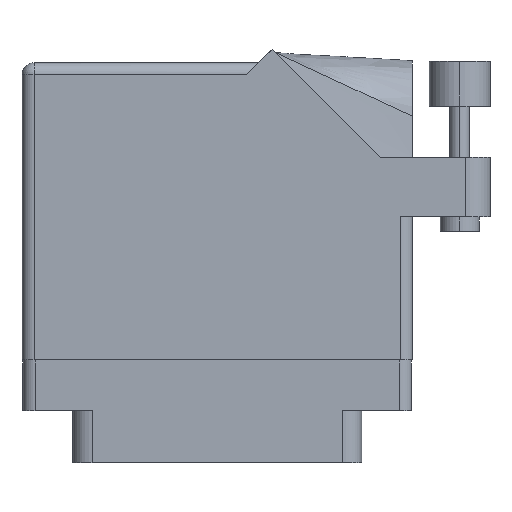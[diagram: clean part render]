
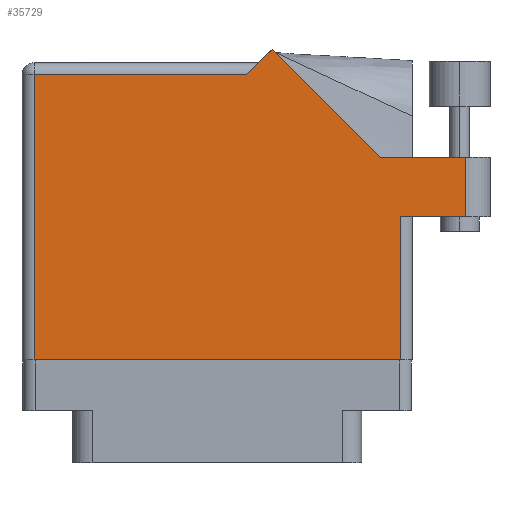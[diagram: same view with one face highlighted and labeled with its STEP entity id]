
A CAD part, front view. The second image highlights one B-rep face of the part: STEP entity #35729.
In plain terms, the highlighted face is planar.
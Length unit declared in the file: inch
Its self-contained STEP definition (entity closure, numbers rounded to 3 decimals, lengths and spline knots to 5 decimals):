
#113 = CARTESIAN_POINT ( 'NONE',  ( 1.155, 1.468, 0. ) ) ;
#852 = DIRECTION ( 'NONE',  ( -1., 0., 0. ) ) ;
#996 = VECTOR ( 'NONE', #35582, 39.37008 ) ;
#2081 = VERTEX_POINT ( 'NONE', #23237 ) ;
#4192 = CARTESIAN_POINT ( 'NONE',  ( 0.062, 0., 0. ) ) ;
#5016 = LINE ( 'NONE', #26424, #30380 ) ;
#5567 = FACE_OUTER_BOUND ( 'NONE', #18233, .T. ) ;
#5643 = VERTEX_POINT ( 'NONE', #17618 ) ;
#6016 = DIRECTION ( 'NONE',  ( 1., 0., 0. ) ) ;
#6865 = EDGE_CURVE ( 'NONE', #38539, #15133, #20468, .T. ) ;
#7112 = LINE ( 'NONE', #20522, #996 ) ;
#7306 = ORIENTED_EDGE ( 'NONE', *, *, #39012, .T. ) ;
#7308 = CARTESIAN_POINT ( 'NONE',  ( 0., 1.468, 0. ) ) ;
#10062 = VECTOR ( 'NONE', #11504, 39.37008 ) ;
#10994 = VECTOR ( 'NONE', #18416, 39.37008 ) ;
#11504 = DIRECTION ( 'NONE',  ( -1., 0., 0. ) ) ;
#12870 = PLANE ( 'NONE',  #25486 ) ;
#13401 = DIRECTION ( 'NONE',  ( -1., 0., 0. ) ) ;
#13534 = DIRECTION ( 'NONE',  ( 0., -1., 0. ) ) ;
#13855 = EDGE_CURVE ( 'NONE', #22827, #17583, #17611, .T. ) ;
#14424 = LINE ( 'NONE', #21102, #37452 ) ;
#14647 = CARTESIAN_POINT ( 'NONE',  ( 1.84442, 1.044, 0. ) ) ;
#15133 = VERTEX_POINT ( 'NONE', #15189 ) ;
#15152 = VERTEX_POINT ( 'NONE', #24652 ) ;
#15189 = CARTESIAN_POINT ( 'NONE',  ( 0.062, 1.468, 0. ) ) ;
#15533 = DIRECTION ( 'NONE',  ( -0.707, -0.707, 0. ) ) ;
#15755 = DIRECTION ( 'NONE',  ( 0., 0., -1. ) ) ;
#16479 = ORIENTED_EDGE ( 'NONE', *, *, #21124, .T. ) ;
#16644 = CARTESIAN_POINT ( 'NONE',  ( 0.062, 0., 0. ) ) ;
#16723 = ORIENTED_EDGE ( 'NONE', *, *, #30208, .T. ) ;
#17583 = VERTEX_POINT ( 'NONE', #34333 ) ;
#17611 = LINE ( 'NONE', #14647, #19009 ) ;
#17618 = CARTESIAN_POINT ( 'NONE',  ( 1.948, 0.737, 0. ) ) ;
#18092 = LINE ( 'NONE', #27018, #10062 ) ;
#18233 = EDGE_LOOP ( 'NONE', ( #26630, #31312, #35486, #31763, #30760, #18553, #16479, #7306, #16723 ) ) ;
#18416 = DIRECTION ( 'NONE',  ( 0., 1., 0. ) ) ;
#18553 = ORIENTED_EDGE ( 'NONE', *, *, #6865, .T. ) ;
#18934 = CARTESIAN_POINT ( 'NONE',  ( 0., 1.53, 0. ) ) ;
#19009 = VECTOR ( 'NONE', #26864, 39.37008 ) ;
#20416 = LINE ( 'NONE', #16644, #27446 ) ;
#20428 = VECTOR ( 'NONE', #6016, 39.37008 ) ;
#20468 = LINE ( 'NONE', #7308, #26105 ) ;
#20522 = CARTESIAN_POINT ( 'NONE',  ( 2.01, 0.737, 0. ) ) ;
#20793 = EDGE_CURVE ( 'NONE', #2081, #26929, #29796, .T. ) ;
#21014 = CARTESIAN_POINT ( 'NONE',  ( 1.84442, 1.044, 0. ) ) ;
#21102 = CARTESIAN_POINT ( 'NONE',  ( 1.217, 1.53, 0. ) ) ;
#21124 = EDGE_CURVE ( 'NONE', #15133, #26565, #20416, .T. ) ;
#22827 = VERTEX_POINT ( 'NONE', #21014 ) ;
#23237 = CARTESIAN_POINT ( 'NONE',  ( 2.285, 0.737, 0. ) ) ;
#24652 = CARTESIAN_POINT ( 'NONE',  ( 1.948, 0., 0. ) ) ;
#25486 = AXIS2_PLACEMENT_3D ( 'NONE', #18934, #15755, #852 ) ;
#26105 = VECTOR ( 'NONE', #13401, 39.37008 ) ;
#26334 = EDGE_CURVE ( 'NONE', #17583, #38539, #14424, .T. ) ;
#26424 = CARTESIAN_POINT ( 'NONE',  ( 1.948, 0.737, 0. ) ) ;
#26565 = VERTEX_POINT ( 'NONE', #4192 ) ;
#26630 = ORIENTED_EDGE ( 'NONE', *, *, #33691, .T. ) ;
#26864 = DIRECTION ( 'NONE',  ( -0.707, 0.707, 0. ) ) ;
#26929 = VERTEX_POINT ( 'NONE', #34815 ) ;
#27018 = CARTESIAN_POINT ( 'NONE',  ( 2.41, 1.044, 0. ) ) ;
#27446 = VECTOR ( 'NONE', #13534, 39.37008 ) ;
#29796 = LINE ( 'NONE', #36930, #10994 ) ;
#30208 = EDGE_CURVE ( 'NONE', #15152, #5643, #5016, .T. ) ;
#30380 = VECTOR ( 'NONE', #38347, 39.37008 ) ;
#30760 = ORIENTED_EDGE ( 'NONE', *, *, #26334, .T. ) ;
#31312 = ORIENTED_EDGE ( 'NONE', *, *, #20793, .T. ) ;
#31763 = ORIENTED_EDGE ( 'NONE', *, *, #13855, .T. ) ;
#32745 = CARTESIAN_POINT ( 'NONE',  ( 0., 0., 0. ) ) ;
#33691 = EDGE_CURVE ( 'NONE', #5643, #2081, #7112, .T. ) ;
#34333 = CARTESIAN_POINT ( 'NONE',  ( 1.28771, 1.60071, 0. ) ) ;
#34497 = LINE ( 'NONE', #32745, #20428 ) ;
#34815 = CARTESIAN_POINT ( 'NONE',  ( 2.285, 1.044, 0. ) ) ;
#35486 = ORIENTED_EDGE ( 'NONE', *, *, #38385, .T. ) ;
#35582 = DIRECTION ( 'NONE',  ( 1., 0., 0. ) ) ;
#35729 = ADVANCED_FACE ( 'NONE', ( #5567 ), #12870, .F. ) ;
#36930 = CARTESIAN_POINT ( 'NONE',  ( 2.285, 1.044, 0. ) ) ;
#37452 = VECTOR ( 'NONE', #15533, 39.37008 ) ;
#38347 = DIRECTION ( 'NONE',  ( 0., 1., 0. ) ) ;
#38385 = EDGE_CURVE ( 'NONE', #26929, #22827, #18092, .T. ) ;
#38539 = VERTEX_POINT ( 'NONE', #113 ) ;
#39012 = EDGE_CURVE ( 'NONE', #26565, #15152, #34497, .T. ) ;
